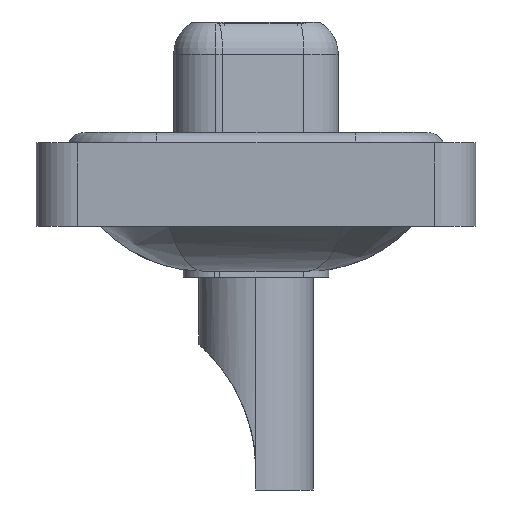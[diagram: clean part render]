
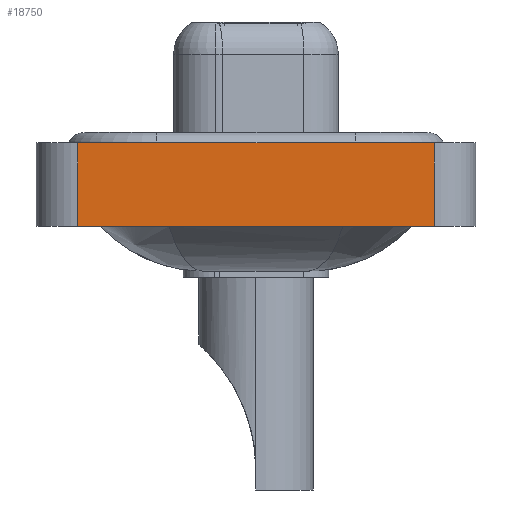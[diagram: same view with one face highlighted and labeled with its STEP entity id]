
A CAD part, left-side view. The second image highlights one B-rep face of the part: STEP entity #18750.
In plain terms, the highlighted planar face has unit normal (-1, 0, 0).
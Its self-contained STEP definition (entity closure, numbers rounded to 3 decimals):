
#261 = CARTESIAN_POINT ( 'NONE',  ( -7.3, -8.55, 0.4 ) ) ;
#516 = DIRECTION ( 'NONE',  ( 0., 0., 1. ) ) ;
#1004 = VECTOR ( 'NONE', #8186, 1000. ) ;
#2876 = EDGE_CURVE ( 'NONE', #16064, #11515, #17263, .T. ) ;
#4328 = CARTESIAN_POINT ( 'NONE',  ( -7.3, -8.55, 0.4 ) ) ;
#4785 = LINE ( 'NONE', #7889, #1004 ) ;
#5833 = EDGE_LOOP ( 'NONE', ( #6221, #9096, #6784, #19587 ) ) ;
#6221 = ORIENTED_EDGE ( 'NONE', *, *, #19066, .T. ) ;
#6784 = ORIENTED_EDGE ( 'NONE', *, *, #2876, .F. ) ;
#6850 = EDGE_CURVE ( 'NONE', #16064, #8958, #4785, .T. ) ;
#7270 = VECTOR ( 'NONE', #14686, 1000. ) ;
#7889 = CARTESIAN_POINT ( 'NONE',  ( -7.3, -8.55, -3.6 ) ) ;
#8186 = DIRECTION ( 'NONE',  ( 0., -1., 0. ) ) ;
#8330 = LINE ( 'NONE', #261, #7270 ) ;
#8958 = VERTEX_POINT ( 'NONE', #11681 ) ;
#9025 = FACE_OUTER_BOUND ( 'NONE', #5833, .T. ) ;
#9096 = ORIENTED_EDGE ( 'NONE', *, *, #17165, .F. ) ;
#10519 = CARTESIAN_POINT ( 'NONE',  ( -7.3, 8.55, -3.6 ) ) ;
#10711 = AXIS2_PLACEMENT_3D ( 'NONE', #17040, #11664, #16839 ) ;
#11515 = VERTEX_POINT ( 'NONE', #17651 ) ;
#11664 = DIRECTION ( 'NONE',  ( -1., 0., 0. ) ) ;
#11681 = CARTESIAN_POINT ( 'NONE',  ( -7.3, -8.55, -3.6 ) ) ;
#12677 = DIRECTION ( 'NONE',  ( 0., 0., 1. ) ) ;
#13291 = CARTESIAN_POINT ( 'NONE',  ( -7.3, -8.55, -3.6 ) ) ;
#14686 = DIRECTION ( 'NONE',  ( 0., -1., 0. ) ) ;
#14794 = PLANE ( 'NONE',  #10711 ) ;
#14848 = LINE ( 'NONE', #13291, #15709 ) ;
#15709 = VECTOR ( 'NONE', #516, 1000. ) ;
#16064 = VERTEX_POINT ( 'NONE', #10519 ) ;
#16781 = VECTOR ( 'NONE', #12677, 1000. ) ;
#16839 = DIRECTION ( 'NONE',  ( 0., 0., 1. ) ) ;
#17040 = CARTESIAN_POINT ( 'NONE',  ( -7.3, -8.55, -3.6 ) ) ;
#17165 = EDGE_CURVE ( 'NONE', #11515, #18392, #8330, .T. ) ;
#17263 = LINE ( 'NONE', #19329, #16781 ) ;
#17651 = CARTESIAN_POINT ( 'NONE',  ( -7.3, 8.55, 0.4 ) ) ;
#18392 = VERTEX_POINT ( 'NONE', #4328 ) ;
#18750 = ADVANCED_FACE ( 'NONE', ( #9025 ), #14794, .T. ) ;
#19066 = EDGE_CURVE ( 'NONE', #8958, #18392, #14848, .T. ) ;
#19329 = CARTESIAN_POINT ( 'NONE',  ( -7.3, 8.55, -3.6 ) ) ;
#19587 = ORIENTED_EDGE ( 'NONE', *, *, #6850, .T. ) ;
